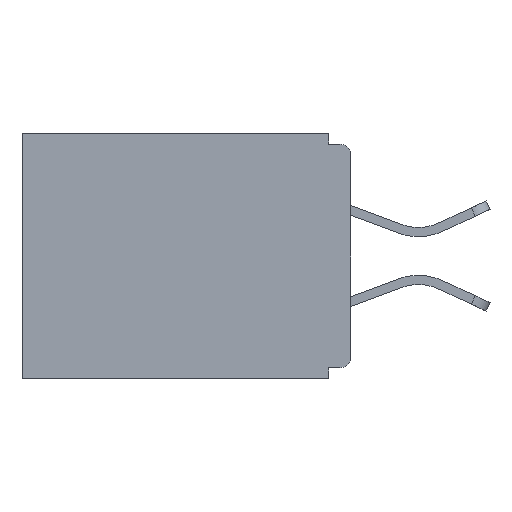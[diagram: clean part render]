
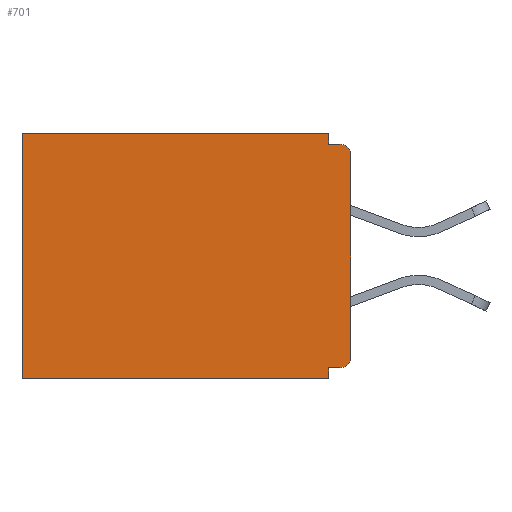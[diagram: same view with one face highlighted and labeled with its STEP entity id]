
A CAD part, left-side view. The second image highlights one B-rep face of the part: STEP entity #701.
In plain terms, the highlighted planar face has unit normal (-1, 0, 0).
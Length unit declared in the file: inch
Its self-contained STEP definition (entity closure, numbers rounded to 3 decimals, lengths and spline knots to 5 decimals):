
#260 = CARTESIAN_POINT ( 'NONE',  ( 0.298, 0.015, -0.03 ) ) ;
#701 = ADVANCED_FACE ( 'NONE', ( #6328 ), #21839, .F. ) ;
#1142 = DIRECTION ( 'NONE',  ( 0., 1., 0. ) ) ;
#1622 = DIRECTION ( 'NONE',  ( 0., 0., -1. ) ) ;
#1781 = EDGE_CURVE ( 'NONE', #19183, #20937, #21024, .T. ) ;
#1829 = ORIENTED_EDGE ( 'NONE', *, *, #14350, .T. ) ;
#2359 = DIRECTION ( 'NONE',  ( 0., 0., -1. ) ) ;
#2396 = DIRECTION ( 'NONE',  ( 0., 0., -1. ) ) ;
#2628 = CARTESIAN_POINT ( 'NONE',  ( 0.298, 0.46, -0.343 ) ) ;
#2770 = CARTESIAN_POINT ( 'NONE',  ( 0.298, 0.46, 0. ) ) ;
#2925 = VECTOR ( 'NONE', #1622, 39.37008 ) ;
#2988 = VECTOR ( 'NONE', #9970, 39.37008 ) ;
#2999 = VERTEX_POINT ( 'NONE', #2628 ) ;
#3022 = DIRECTION ( 'NONE',  ( -1., 0., 0. ) ) ;
#3028 = CARTESIAN_POINT ( 'NONE',  ( 0.298, 0.015, -0.328 ) ) ;
#3538 = EDGE_LOOP ( 'NONE', ( #15161, #5069, #9084, #21530, #5893, #16343, #7967, #3756, #1829, #5725 ) ) ;
#3756 = ORIENTED_EDGE ( 'NONE', *, *, #9147, .F. ) ;
#3849 = CARTESIAN_POINT ( 'NONE',  ( 0.298, 0.015, -0.015 ) ) ;
#5069 = ORIENTED_EDGE ( 'NONE', *, *, #1781, .F. ) ;
#5304 = CARTESIAN_POINT ( 'NONE',  ( 0.298, 0., 0. ) ) ;
#5595 = VECTOR ( 'NONE', #9245, 39.37008 ) ;
#5725 = ORIENTED_EDGE ( 'NONE', *, *, #14983, .F. ) ;
#5893 = ORIENTED_EDGE ( 'NONE', *, *, #19401, .T. ) ;
#5929 = LINE ( 'NONE', #2770, #5595 ) ;
#6328 = FACE_OUTER_BOUND ( 'NONE', #3538, .T. ) ;
#6685 = VERTEX_POINT ( 'NONE', #24253 ) ;
#6711 = CARTESIAN_POINT ( 'NONE',  ( 0.298, 0., -0.03 ) ) ;
#7053 = VECTOR ( 'NONE', #2359, 39.37008 ) ;
#7692 = VECTOR ( 'NONE', #1142, 39.37008 ) ;
#7967 = ORIENTED_EDGE ( 'NONE', *, *, #20769, .F. ) ;
#9084 = ORIENTED_EDGE ( 'NONE', *, *, #26716, .F. ) ;
#9147 = EDGE_CURVE ( 'NONE', #13699, #22370, #19721, .T. ) ;
#9245 = DIRECTION ( 'NONE',  ( 0., 0., -1. ) ) ;
#9357 = EDGE_CURVE ( 'NONE', #9951, #2999, #14137, .T. ) ;
#9387 = DIRECTION ( 'NONE',  ( 1., 0., 0. ) ) ;
#9838 = VERTEX_POINT ( 'NONE', #12556 ) ;
#9951 = VERTEX_POINT ( 'NONE', #15779 ) ;
#9970 = DIRECTION ( 'NONE',  ( 0., 1., 0. ) ) ;
#10368 = AXIS2_PLACEMENT_3D ( 'NONE', #19840, #9387, #13734 ) ;
#10929 = CARTESIAN_POINT ( 'NONE',  ( 0.298, 0., -0.015 ) ) ;
#12556 = CARTESIAN_POINT ( 'NONE',  ( 0.298, 0., -0.313 ) ) ;
#12620 = EDGE_CURVE ( 'NONE', #25591, #6685, #25108, .T. ) ;
#12780 = VECTOR ( 'NONE', #15902, 39.37008 ) ;
#12847 = DIRECTION ( 'NONE',  ( 0., -1., 0. ) ) ;
#12901 = CIRCLE ( 'NONE', #27160, 0.015 ) ;
#13098 = DIRECTION ( 'NONE',  ( 0., 1., 0. ) ) ;
#13699 = VERTEX_POINT ( 'NONE', #3028 ) ;
#13734 = DIRECTION ( 'NONE',  ( 0., 0., -1. ) ) ;
#14137 = LINE ( 'NONE', #20307, #2988 ) ;
#14165 = VECTOR ( 'NONE', #13098, 39.37008 ) ;
#14350 = EDGE_CURVE ( 'NONE', #13699, #9838, #12901, .T. ) ;
#14757 = AXIS2_PLACEMENT_3D ( 'NONE', #260, #14978, #2396 ) ;
#14851 = CARTESIAN_POINT ( 'NONE',  ( 0.298, 0.031, -0.343 ) ) ;
#14978 = DIRECTION ( 'NONE',  ( -1., 0., 0. ) ) ;
#14983 = EDGE_CURVE ( 'NONE', #24309, #9838, #18314, .T. ) ;
#15161 = ORIENTED_EDGE ( 'NONE', *, *, #26369, .T. ) ;
#15779 = CARTESIAN_POINT ( 'NONE',  ( 0.298, 0.031, -0.343 ) ) ;
#15902 = DIRECTION ( 'NONE',  ( 0., 0., -1. ) ) ;
#15983 = LINE ( 'NONE', #14851, #7053 ) ;
#16343 = ORIENTED_EDGE ( 'NONE', *, *, #9357, .F. ) ;
#16946 = CARTESIAN_POINT ( 'NONE',  ( 0.298, 0.015, -0.313 ) ) ;
#18314 = LINE ( 'NONE', #26707, #2925 ) ;
#19183 = VERTEX_POINT ( 'NONE', #25852 ) ;
#19401 = EDGE_CURVE ( 'NONE', #6685, #2999, #5929, .T. ) ;
#19624 = CARTESIAN_POINT ( 'NONE',  ( 0.298, 0.031, 0. ) ) ;
#19721 = LINE ( 'NONE', #19768, #14165 ) ;
#19768 = CARTESIAN_POINT ( 'NONE',  ( 0.298, 0., -0.328 ) ) ;
#19840 = CARTESIAN_POINT ( 'NONE',  ( 0.298, 0., 0. ) ) ;
#20307 = CARTESIAN_POINT ( 'NONE',  ( 0.298, 0., -0.343 ) ) ;
#20769 = EDGE_CURVE ( 'NONE', #22370, #9951, #26540, .T. ) ;
#20937 = VERTEX_POINT ( 'NONE', #3849 ) ;
#21024 = LINE ( 'NONE', #10929, #23005 ) ;
#21530 = ORIENTED_EDGE ( 'NONE', *, *, #12620, .T. ) ;
#21839 = PLANE ( 'NONE',  #10368 ) ;
#22370 = VERTEX_POINT ( 'NONE', #26083 ) ;
#23005 = VECTOR ( 'NONE', #12847, 39.37008 ) ;
#23627 = DIRECTION ( 'NONE',  ( 0., 0., -1. ) ) ;
#24253 = CARTESIAN_POINT ( 'NONE',  ( 0.298, 0.46, 0. ) ) ;
#24286 = CARTESIAN_POINT ( 'NONE',  ( 0.298, 0.031, -0.343 ) ) ;
#24309 = VERTEX_POINT ( 'NONE', #6711 ) ;
#25108 = LINE ( 'NONE', #5304, #7692 ) ;
#25591 = VERTEX_POINT ( 'NONE', #19624 ) ;
#25852 = CARTESIAN_POINT ( 'NONE',  ( 0.298, 0.031, -0.015 ) ) ;
#26083 = CARTESIAN_POINT ( 'NONE',  ( 0.298, 0.031, -0.328 ) ) ;
#26369 = EDGE_CURVE ( 'NONE', #24309, #20937, #27096, .T. ) ;
#26540 = LINE ( 'NONE', #24286, #12780 ) ;
#26707 = CARTESIAN_POINT ( 'NONE',  ( 0.298, 0., 0. ) ) ;
#26716 = EDGE_CURVE ( 'NONE', #25591, #19183, #15983, .T. ) ;
#27096 = CIRCLE ( 'NONE', #14757, 0.015 ) ;
#27160 = AXIS2_PLACEMENT_3D ( 'NONE', #16946, #3022, #23627 ) ;
